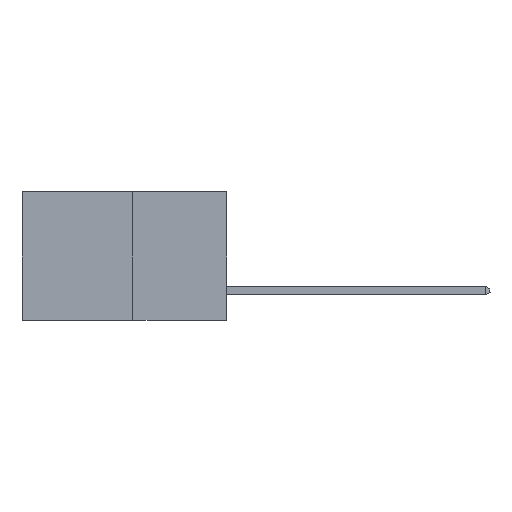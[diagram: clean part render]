
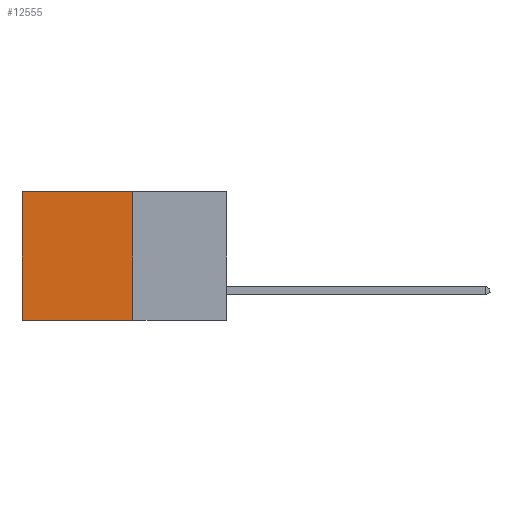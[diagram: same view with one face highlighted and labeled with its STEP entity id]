
A CAD part, left-side view. The second image highlights one B-rep face of the part: STEP entity #12555.
In plain terms, the highlighted planar face has unit normal (-1, 0, 0).
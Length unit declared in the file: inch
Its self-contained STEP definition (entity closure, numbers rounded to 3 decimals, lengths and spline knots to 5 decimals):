
#1853 = LINE ( 'NONE', #13167, #24957 ) ;
#2391 = LINE ( 'NONE', #9769, #25500 ) ;
#5025 = AXIS2_PLACEMENT_3D ( 'NONE', #12778, #12773, #12738 ) ;
#5982 = EDGE_CURVE ( 'NONE', #7929, #14609, #1853, .T. ) ;
#6195 = CARTESIAN_POINT ( 'NONE',  ( 0.277, 0.27, -0.37 ) ) ;
#6477 = EDGE_CURVE ( 'NONE', #14609, #10862, #12229, .T. ) ;
#6998 = FACE_OUTER_BOUND ( 'NONE', #16810, .T. ) ;
#7929 = VERTEX_POINT ( 'NONE', #8477 ) ;
#8477 = CARTESIAN_POINT ( 'NONE',  ( 0.277, 0.27, 0. ) ) ;
#9769 = CARTESIAN_POINT ( 'NONE',  ( 0.277, 0.59, -0.37 ) ) ;
#9831 = CARTESIAN_POINT ( 'NONE',  ( 0.277, 0.27, 0. ) ) ;
#10144 = EDGE_CURVE ( 'NONE', #7929, #17161, #22604, .T. ) ;
#10862 = VERTEX_POINT ( 'NONE', #15385 ) ;
#12229 = LINE ( 'NONE', #20315, #18216 ) ;
#12555 = ADVANCED_FACE ( 'NONE', ( #6998 ), #12838, .F. ) ;
#12738 = DIRECTION ( 'NONE',  ( 0., 0., -1. ) ) ;
#12773 = DIRECTION ( 'NONE',  ( 1., 0., 0. ) ) ;
#12778 = CARTESIAN_POINT ( 'NONE',  ( 0.277, 0.27, -0.37 ) ) ;
#12838 = PLANE ( 'NONE',  #5025 ) ;
#13167 = CARTESIAN_POINT ( 'NONE',  ( 0.277, 0.27, -0.37 ) ) ;
#13597 = ORIENTED_EDGE ( 'NONE', *, *, #5982, .F. ) ;
#14532 = DIRECTION ( 'NONE',  ( 0., 1., 0. ) ) ;
#14609 = VERTEX_POINT ( 'NONE', #6195 ) ;
#15146 = CARTESIAN_POINT ( 'NONE',  ( 0.277, 0.59, 0. ) ) ;
#15385 = CARTESIAN_POINT ( 'NONE',  ( 0.277, 0.59, -0.37 ) ) ;
#16810 = EDGE_LOOP ( 'NONE', ( #17300, #24650, #13597, #17098 ) ) ;
#17098 = ORIENTED_EDGE ( 'NONE', *, *, #10144, .T. ) ;
#17161 = VERTEX_POINT ( 'NONE', #15146 ) ;
#17300 = ORIENTED_EDGE ( 'NONE', *, *, #23945, .T. ) ;
#18216 = VECTOR ( 'NONE', #14532, 39.37008 ) ;
#20279 = DIRECTION ( 'NONE',  ( 0., 0., -1. ) ) ;
#20315 = CARTESIAN_POINT ( 'NONE',  ( 0.277, 0.27, -0.37 ) ) ;
#20932 = DIRECTION ( 'NONE',  ( 0., 1., 0. ) ) ;
#21898 = VECTOR ( 'NONE', #20932, 39.37008 ) ;
#22604 = LINE ( 'NONE', #9831, #21898 ) ;
#23945 = EDGE_CURVE ( 'NONE', #17161, #10862, #2391, .T. ) ;
#24650 = ORIENTED_EDGE ( 'NONE', *, *, #6477, .F. ) ;
#24957 = VECTOR ( 'NONE', #20279, 39.37008 ) ;
#25500 = VECTOR ( 'NONE', #27736, 39.37008 ) ;
#27736 = DIRECTION ( 'NONE',  ( 0., 0., -1. ) ) ;
